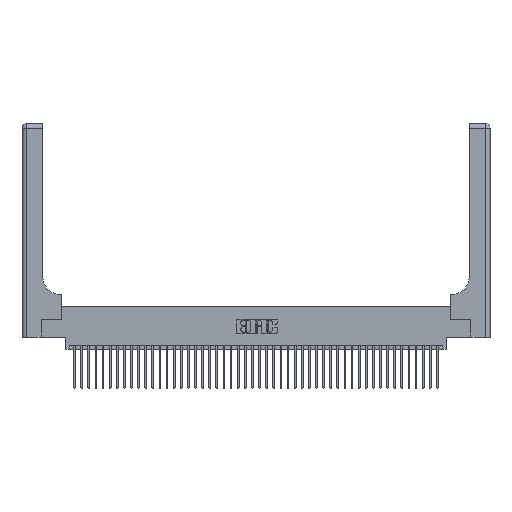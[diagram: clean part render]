
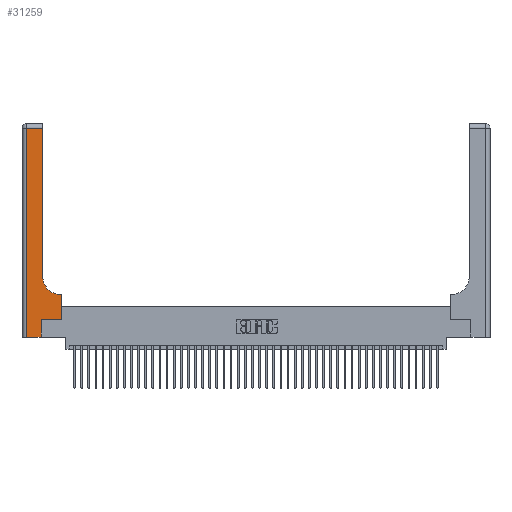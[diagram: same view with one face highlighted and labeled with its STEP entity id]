
A CAD part, top view. The second image highlights one B-rep face of the part: STEP entity #31259.
In plain terms, the highlighted planar face has unit normal (0, 0, 1).
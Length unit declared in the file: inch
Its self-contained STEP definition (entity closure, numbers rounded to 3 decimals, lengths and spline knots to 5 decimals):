
#407 = ORIENTED_EDGE ( 'NONE', *, *, #35488, .T. ) ;
#739 = VECTOR ( 'NONE', #32837, 39.37008 ) ;
#770 = ORIENTED_EDGE ( 'NONE', *, *, #20508, .T. ) ;
#969 = LINE ( 'NONE', #18396, #38887 ) ;
#1260 = CARTESIAN_POINT ( 'NONE',  ( 0.269, 0.25, 0.37 ) ) ;
#1554 = LINE ( 'NONE', #40738, #21050 ) ;
#2414 = ORIENTED_EDGE ( 'NONE', *, *, #11349, .T. ) ;
#2661 = EDGE_CURVE ( 'NONE', #8646, #2865, #21953, .T. ) ;
#2683 = VECTOR ( 'NONE', #42967, 39.37008 ) ;
#2865 = VERTEX_POINT ( 'NONE', #8167 ) ;
#4627 = LINE ( 'NONE', #41129, #38693 ) ;
#4677 = AXIS2_PLACEMENT_3D ( 'NONE', #18241, #14256, #38654 ) ;
#6096 = CARTESIAN_POINT ( 'NONE',  ( 0.2915, 0.85, 0.37 ) ) ;
#6194 = VECTOR ( 'NONE', #12309, 39.37008 ) ;
#8056 = ORIENTED_EDGE ( 'NONE', *, *, #2661, .T. ) ;
#8160 = ORIENTED_EDGE ( 'NONE', *, *, #25372, .T. ) ;
#8167 = CARTESIAN_POINT ( 'NONE',  ( 0.2915, 2.94, 0.37 ) ) ;
#8462 = ORIENTED_EDGE ( 'NONE', *, *, #11215, .T. ) ;
#8646 = VERTEX_POINT ( 'NONE', #6096 ) ;
#9983 = CARTESIAN_POINT ( 'NONE',  ( 0.06, 0., 0.37 ) ) ;
#11215 = EDGE_CURVE ( 'NONE', #19469, #31500, #15410, .T. ) ;
#11349 = EDGE_CURVE ( 'NONE', #36446, #30389, #19235, .T. ) ;
#11692 = DIRECTION ( 'NONE',  ( 1., 0., 0. ) ) ;
#12309 = DIRECTION ( 'NONE',  ( 0., 1., 0. ) ) ;
#12883 = CARTESIAN_POINT ( 'NONE',  ( 0.5585, 0.25, 0.37 ) ) ;
#13211 = VECTOR ( 'NONE', #18440, 39.37008 ) ;
#14145 = CARTESIAN_POINT ( 'NONE',  ( 0.5585, 0.25, 0.37 ) ) ;
#14256 = DIRECTION ( 'NONE',  ( 0., 0., -1. ) ) ;
#14903 = CARTESIAN_POINT ( 'NONE',  ( 0.06, 2.94, 0.37 ) ) ;
#15410 = LINE ( 'NONE', #12883, #6194 ) ;
#16317 = CARTESIAN_POINT ( 'NONE',  ( 0.2915, 3., 0.37 ) ) ;
#16807 = DIRECTION ( 'NONE',  ( 1., 0., 0. ) ) ;
#18241 = CARTESIAN_POINT ( 'NONE',  ( 0., 3., 0.37 ) ) ;
#18353 = CARTESIAN_POINT ( 'NONE',  ( 0.269, 0., 0.37 ) ) ;
#18396 = CARTESIAN_POINT ( 'NONE',  ( 0.269, 0.25, 0.37 ) ) ;
#18440 = DIRECTION ( 'NONE',  ( 0., 1., 0. ) ) ;
#19002 = ORIENTED_EDGE ( 'NONE', *, *, #30692, .T. ) ;
#19235 = LINE ( 'NONE', #25278, #739 ) ;
#19469 = VERTEX_POINT ( 'NONE', #14145 ) ;
#20051 = LINE ( 'NONE', #42803, #2683 ) ;
#20508 = EDGE_CURVE ( 'NONE', #38780, #35098, #4627, .T. ) ;
#21050 = VECTOR ( 'NONE', #44532, 39.37008 ) ;
#21064 = ORIENTED_EDGE ( 'NONE', *, *, #33709, .T. ) ;
#21953 = LINE ( 'NONE', #16317, #13211 ) ;
#22784 = AXIS2_PLACEMENT_3D ( 'NONE', #28450, #31914, #35416 ) ;
#25278 = CARTESIAN_POINT ( 'NONE',  ( 0.06, 3., 0.37 ) ) ;
#25372 = EDGE_CURVE ( 'NONE', #2865, #36446, #1554, .T. ) ;
#27171 = CARTESIAN_POINT ( 'NONE',  ( 0., 0., 0.37 ) ) ;
#28450 = CARTESIAN_POINT ( 'NONE',  ( 0.5415, 0.85, 0.37 ) ) ;
#30389 = VERTEX_POINT ( 'NONE', #9983 ) ;
#30692 = EDGE_CURVE ( 'NONE', #31500, #39351, #20051, .T. ) ;
#31259 = ADVANCED_FACE ( 'NONE', ( #36826 ), #31412, .F. ) ;
#31412 = PLANE ( 'NONE',  #4677 ) ;
#31425 = EDGE_CURVE ( 'NONE', #35098, #19469, #969, .T. ) ;
#31500 = VERTEX_POINT ( 'NONE', #40847 ) ;
#31914 = DIRECTION ( 'NONE',  ( 0., 0., -1. ) ) ;
#32837 = DIRECTION ( 'NONE',  ( 0., -1., 0. ) ) ;
#33709 = EDGE_CURVE ( 'NONE', #39351, #8646, #36195, .T. ) ;
#35098 = VERTEX_POINT ( 'NONE', #1260 ) ;
#35416 = DIRECTION ( 'NONE',  ( 1., 0., 0. ) ) ;
#35488 = EDGE_CURVE ( 'NONE', #30389, #38780, #36053, .T. ) ;
#35744 = ORIENTED_EDGE ( 'NONE', *, *, #31425, .T. ) ;
#36053 = LINE ( 'NONE', #27171, #41862 ) ;
#36195 = CIRCLE ( 'NONE', #22784, 0.25 ) ;
#36446 = VERTEX_POINT ( 'NONE', #14903 ) ;
#36826 = FACE_OUTER_BOUND ( 'NONE', #43975, .T. ) ;
#38007 = CARTESIAN_POINT ( 'NONE',  ( 0.5415, 0.6, 0.37 ) ) ;
#38654 = DIRECTION ( 'NONE',  ( -1., 0., 0. ) ) ;
#38693 = VECTOR ( 'NONE', #44772, 39.37008 ) ;
#38780 = VERTEX_POINT ( 'NONE', #18353 ) ;
#38887 = VECTOR ( 'NONE', #11692, 39.37008 ) ;
#39351 = VERTEX_POINT ( 'NONE', #38007 ) ;
#40738 = CARTESIAN_POINT ( 'NONE',  ( 0., 2.94, 0.37 ) ) ;
#40847 = CARTESIAN_POINT ( 'NONE',  ( 0.5585, 0.6, 0.37 ) ) ;
#41129 = CARTESIAN_POINT ( 'NONE',  ( 0.269, 0., 0.37 ) ) ;
#41862 = VECTOR ( 'NONE', #16807, 39.37008 ) ;
#42803 = CARTESIAN_POINT ( 'NONE',  ( 0.2915, 0.6, 0.37 ) ) ;
#42967 = DIRECTION ( 'NONE',  ( -1., 0., 0. ) ) ;
#43975 = EDGE_LOOP ( 'NONE', ( #8056, #8160, #2414, #407, #770, #35744, #8462, #19002, #21064 ) ) ;
#44532 = DIRECTION ( 'NONE',  ( -1., 0., 0. ) ) ;
#44772 = DIRECTION ( 'NONE',  ( 0., 1., 0. ) ) ;
